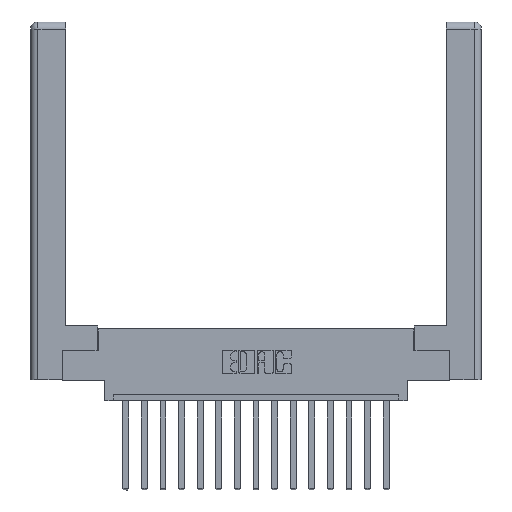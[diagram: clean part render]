
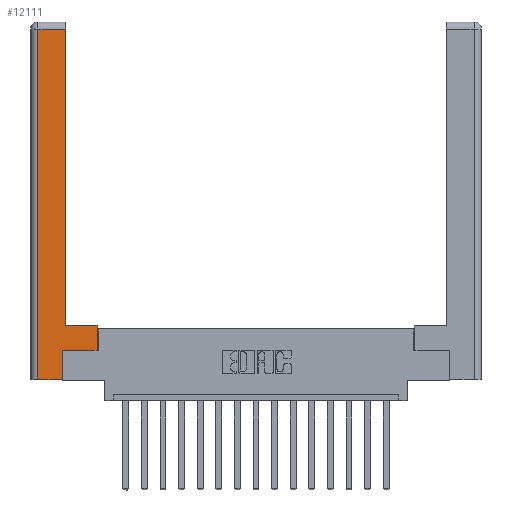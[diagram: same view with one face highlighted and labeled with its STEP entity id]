
A CAD part, top view. The second image highlights one B-rep face of the part: STEP entity #12111.
In plain terms, the highlighted planar face has unit normal (0, 0, 1).
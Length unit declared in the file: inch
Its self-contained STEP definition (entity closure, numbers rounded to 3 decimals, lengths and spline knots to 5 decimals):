
#428 = LINE ( 'NONE', #7800, #828 ) ;
#828 = VECTOR ( 'NONE', #6541, 39.37008 ) ;
#1207 = CARTESIAN_POINT ( 'NONE',  ( 0.565, 0.245, 0. ) ) ;
#1362 = VECTOR ( 'NONE', #15854, 39.37008 ) ;
#1680 = VECTOR ( 'NONE', #8752, 39.37008 ) ;
#1873 = DIRECTION ( 'NONE',  ( 0., 1., 0. ) ) ;
#1920 = CARTESIAN_POINT ( 'NONE',  ( 0.0615, 2.94, 0. ) ) ;
#2436 = DIRECTION ( 'NONE',  ( 1., 0., 0. ) ) ;
#3122 = DIRECTION ( 'NONE',  ( 0., 0., -1. ) ) ;
#3177 = DIRECTION ( 'NONE',  ( -1., 0., 0. ) ) ;
#3828 = VERTEX_POINT ( 'NONE', #14044 ) ;
#4055 = CARTESIAN_POINT ( 'NONE',  ( 0.295, 0.45, 0. ) ) ;
#4787 = ORIENTED_EDGE ( 'NONE', *, *, #15535, .T. ) ;
#4960 = CARTESIAN_POINT ( 'NONE',  ( 0.265, 0.245, 0. ) ) ;
#5030 = ORIENTED_EDGE ( 'NONE', *, *, #6212, .T. ) ;
#5101 = LINE ( 'NONE', #1920, #5299 ) ;
#5186 = LINE ( 'NONE', #7396, #1680 ) ;
#5214 = EDGE_LOOP ( 'NONE', ( #9284, #7971, #10527, #6166, #6219, #9780, #4787, #5030 ) ) ;
#5299 = VECTOR ( 'NONE', #12488, 39.37008 ) ;
#5809 = VERTEX_POINT ( 'NONE', #15497 ) ;
#6166 = ORIENTED_EDGE ( 'NONE', *, *, #14382, .T. ) ;
#6212 = EDGE_CURVE ( 'NONE', #3828, #6352, #428, .T. ) ;
#6219 = ORIENTED_EDGE ( 'NONE', *, *, #15388, .T. ) ;
#6352 = VERTEX_POINT ( 'NONE', #4055 ) ;
#6541 = DIRECTION ( 'NONE',  ( -1., 0., 0. ) ) ;
#7072 = CARTESIAN_POINT ( 'NONE',  ( 0.565, 0.45, 0. ) ) ;
#7396 = CARTESIAN_POINT ( 'NONE',  ( 0.265, 0., 0. ) ) ;
#7800 = CARTESIAN_POINT ( 'NONE',  ( 0.295, 0.45, 0. ) ) ;
#7971 = ORIENTED_EDGE ( 'NONE', *, *, #8755, .T. ) ;
#8376 = CARTESIAN_POINT ( 'NONE',  ( 0.0615, 0., 0. ) ) ;
#8474 = EDGE_CURVE ( 'NONE', #6352, #5809, #17004, .T. ) ;
#8690 = LINE ( 'NONE', #7072, #13089 ) ;
#8752 = DIRECTION ( 'NONE',  ( 1., 0., 0. ) ) ;
#8755 = EDGE_CURVE ( 'NONE', #5809, #13791, #5101, .T. ) ;
#9219 = DIRECTION ( 'NONE',  ( 0., 1., 0. ) ) ;
#9284 = ORIENTED_EDGE ( 'NONE', *, *, #8474, .T. ) ;
#9368 = VERTEX_POINT ( 'NONE', #4960 ) ;
#9572 = VECTOR ( 'NONE', #2436, 39.37008 ) ;
#9603 = DIRECTION ( 'NONE',  ( 0., 1., 0. ) ) ;
#9728 = PLANE ( 'NONE',  #13282 ) ;
#9780 = ORIENTED_EDGE ( 'NONE', *, *, #13331, .T. ) ;
#9805 = CARTESIAN_POINT ( 'NONE',  ( 0.295, 3., 0. ) ) ;
#9941 = VECTOR ( 'NONE', #9219, 39.37008 ) ;
#10013 = CARTESIAN_POINT ( 'NONE',  ( 0.265, 0., 0. ) ) ;
#10404 = LINE ( 'NONE', #1207, #9572 ) ;
#10527 = ORIENTED_EDGE ( 'NONE', *, *, #11458, .T. ) ;
#10565 = LINE ( 'NONE', #12025, #9941 ) ;
#10949 = CARTESIAN_POINT ( 'NONE',  ( 0., 0., 0. ) ) ;
#11398 = VERTEX_POINT ( 'NONE', #14709 ) ;
#11458 = EDGE_CURVE ( 'NONE', #13791, #13016, #16570, .T. ) ;
#12025 = CARTESIAN_POINT ( 'NONE',  ( 0.265, 0.245, 0. ) ) ;
#12111 = ADVANCED_FACE ( 'NONE', ( #15916 ), #9728, .F. ) ;
#12112 = CARTESIAN_POINT ( 'NONE',  ( 0.0615, 0., 0. ) ) ;
#12488 = DIRECTION ( 'NONE',  ( -1., 0., 0. ) ) ;
#12840 = VECTOR ( 'NONE', #1873, 39.37008 ) ;
#13016 = VERTEX_POINT ( 'NONE', #8376 ) ;
#13089 = VECTOR ( 'NONE', #9603, 39.37008 ) ;
#13282 = AXIS2_PLACEMENT_3D ( 'NONE', #10949, #3122, #3177 ) ;
#13331 = EDGE_CURVE ( 'NONE', #9368, #11398, #10404, .T. ) ;
#13791 = VERTEX_POINT ( 'NONE', #15328 ) ;
#14044 = CARTESIAN_POINT ( 'NONE',  ( 0.565, 0.45, 0. ) ) ;
#14382 = EDGE_CURVE ( 'NONE', #13016, #15248, #5186, .T. ) ;
#14709 = CARTESIAN_POINT ( 'NONE',  ( 0.565, 0.245, 0. ) ) ;
#15248 = VERTEX_POINT ( 'NONE', #10013 ) ;
#15328 = CARTESIAN_POINT ( 'NONE',  ( 0.0615, 2.94, 0. ) ) ;
#15388 = EDGE_CURVE ( 'NONE', #15248, #9368, #10565, .T. ) ;
#15497 = CARTESIAN_POINT ( 'NONE',  ( 0.295, 2.94, 0. ) ) ;
#15535 = EDGE_CURVE ( 'NONE', #11398, #3828, #8690, .T. ) ;
#15854 = DIRECTION ( 'NONE',  ( 0., -1., 0. ) ) ;
#15916 = FACE_OUTER_BOUND ( 'NONE', #5214, .T. ) ;
#16570 = LINE ( 'NONE', #12112, #1362 ) ;
#17004 = LINE ( 'NONE', #9805, #12840 ) ;
